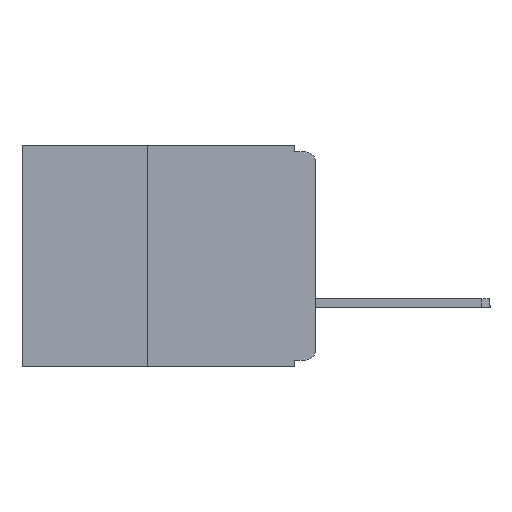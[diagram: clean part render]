
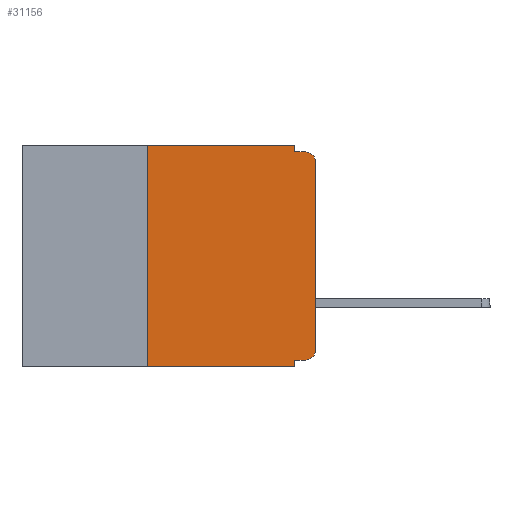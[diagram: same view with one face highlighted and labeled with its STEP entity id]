
A CAD part, left-side view. The second image highlights one B-rep face of the part: STEP entity #31156.
In plain terms, the highlighted planar face has unit normal (-1, 0, 0).
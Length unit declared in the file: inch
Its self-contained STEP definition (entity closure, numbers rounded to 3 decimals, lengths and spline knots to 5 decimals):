
#311 = VERTEX_POINT ( 'NONE', #29264 ) ;
#524 = DIRECTION ( 'NONE',  ( 0., 0., -1. ) ) ;
#1039 = ORIENTED_EDGE ( 'NONE', *, *, #28434, .F. ) ;
#1153 = VECTOR ( 'NONE', #16576, 39.37008 ) ;
#1636 = EDGE_CURVE ( 'NONE', #12275, #311, #32220, .T. ) ;
#1720 = LINE ( 'NONE', #27020, #27956 ) ;
#1995 = DIRECTION ( 'NONE',  ( -1., 0., 0. ) ) ;
#2628 = DIRECTION ( 'NONE',  ( 0., 0., -1. ) ) ;
#2970 = EDGE_CURVE ( 'NONE', #29224, #13932, #3359, .T. ) ;
#3237 = EDGE_CURVE ( 'NONE', #29224, #23874, #23327, .T. ) ;
#3359 = CIRCLE ( 'NONE', #26823, 0.015 ) ;
#4114 = LINE ( 'NONE', #27112, #16819 ) ;
#4340 = DIRECTION ( 'NONE',  ( 0., -1., 0. ) ) ;
#4427 = EDGE_CURVE ( 'NONE', #311, #22659, #15562, .T. ) ;
#4433 = ORIENTED_EDGE ( 'NONE', *, *, #3237, .F. ) ;
#5197 = VERTEX_POINT ( 'NONE', #29304 ) ;
#5385 = VECTOR ( 'NONE', #4340, 39.37008 ) ;
#5845 = CARTESIAN_POINT ( 'NONE',  ( 0., 0.437, 0. ) ) ;
#5871 = EDGE_CURVE ( 'NONE', #24997, #5197, #11295, .T. ) ;
#6599 = LINE ( 'NONE', #30603, #20154 ) ;
#8178 = CARTESIAN_POINT ( 'NONE',  ( 0., 0.25, -0.33 ) ) ;
#8509 = DIRECTION ( 'NONE',  ( 0., 1., 0. ) ) ;
#8709 = AXIS2_PLACEMENT_3D ( 'NONE', #32903, #16724, #524 ) ;
#8939 = VECTOR ( 'NONE', #8509, 39.37008 ) ;
#9753 = CARTESIAN_POINT ( 'NONE',  ( 0., 0.25, -0.33 ) ) ;
#9956 = ORIENTED_EDGE ( 'NONE', *, *, #15061, .T. ) ;
#9985 = ORIENTED_EDGE ( 'NONE', *, *, #2970, .T. ) ;
#11186 = CARTESIAN_POINT ( 'NONE',  ( 0., 0., -0.32 ) ) ;
#11295 = CIRCLE ( 'NONE', #8709, 0.015 ) ;
#12275 = VERTEX_POINT ( 'NONE', #9753 ) ;
#12284 = CARTESIAN_POINT ( 'NONE',  ( 0., 0.031, -0.32 ) ) ;
#12908 = DIRECTION ( 'NONE',  ( 0., -1., 0. ) ) ;
#13334 = ORIENTED_EDGE ( 'NONE', *, *, #4427, .F. ) ;
#13511 = DIRECTION ( 'NONE',  ( 0., 0., -1. ) ) ;
#13932 = VERTEX_POINT ( 'NONE', #15771 ) ;
#14404 = DIRECTION ( 'NONE',  ( 0., 0., 1. ) ) ;
#14422 = DIRECTION ( 'NONE',  ( 0., 0., 1. ) ) ;
#14890 = VERTEX_POINT ( 'NONE', #19896 ) ;
#15061 = EDGE_CURVE ( 'NONE', #12275, #25170, #18935, .T. ) ;
#15562 = LINE ( 'NONE', #5845, #1153 ) ;
#15644 = CARTESIAN_POINT ( 'NONE',  ( 0., 0., -0.025 ) ) ;
#15771 = CARTESIAN_POINT ( 'NONE',  ( 0., 0., -0.305 ) ) ;
#16576 = DIRECTION ( 'NONE',  ( 0., -1., 0. ) ) ;
#16724 = DIRECTION ( 'NONE',  ( -1., 0., 0. ) ) ;
#16819 = VECTOR ( 'NONE', #29806, 39.37008 ) ;
#17506 = VECTOR ( 'NONE', #12908, 39.37008 ) ;
#18240 = CARTESIAN_POINT ( 'NONE',  ( 0., 0.015, -0.305 ) ) ;
#18289 = FACE_OUTER_BOUND ( 'NONE', #19905, .T. ) ;
#18377 = LINE ( 'NONE', #21111, #17506 ) ;
#18566 = ORIENTED_EDGE ( 'NONE', *, *, #21559, .F. ) ;
#18868 = DIRECTION ( 'NONE',  ( 1., 0., 0. ) ) ;
#18935 = LINE ( 'NONE', #20583, #5385 ) ;
#19085 = CARTESIAN_POINT ( 'NONE',  ( 0., 0.031, -0.33 ) ) ;
#19896 = CARTESIAN_POINT ( 'NONE',  ( 0., 0.031, -0.01 ) ) ;
#19905 = EDGE_LOOP ( 'NONE', ( #29741, #32492, #1039, #18566, #13334, #25406, #9956, #29059, #4433, #9985 ) ) ;
#19943 = EDGE_CURVE ( 'NONE', #23874, #25170, #1720, .T. ) ;
#20154 = VECTOR ( 'NONE', #14404, 39.37008 ) ;
#20583 = CARTESIAN_POINT ( 'NONE',  ( 0., 0.437, -0.33 ) ) ;
#20972 = DIRECTION ( 'NONE',  ( 0., 0., -1. ) ) ;
#21111 = CARTESIAN_POINT ( 'NONE',  ( 0., 0., -0.01 ) ) ;
#21559 = EDGE_CURVE ( 'NONE', #22659, #14890, #4114, .T. ) ;
#22659 = VERTEX_POINT ( 'NONE', #34323 ) ;
#23327 = LINE ( 'NONE', #11186, #8939 ) ;
#23874 = VERTEX_POINT ( 'NONE', #12284 ) ;
#24997 = VERTEX_POINT ( 'NONE', #15644 ) ;
#25081 = VECTOR ( 'NONE', #14422, 39.37008 ) ;
#25170 = VERTEX_POINT ( 'NONE', #19085 ) ;
#25406 = ORIENTED_EDGE ( 'NONE', *, *, #1636, .F. ) ;
#26823 = AXIS2_PLACEMENT_3D ( 'NONE', #18240, #1995, #20972 ) ;
#27020 = CARTESIAN_POINT ( 'NONE',  ( 0., 0.031, -0.33 ) ) ;
#27112 = CARTESIAN_POINT ( 'NONE',  ( 0., 0.031, 0. ) ) ;
#27477 = EDGE_CURVE ( 'NONE', #13932, #24997, #6599, .T. ) ;
#27956 = VECTOR ( 'NONE', #13511, 39.37008 ) ;
#28434 = EDGE_CURVE ( 'NONE', #14890, #5197, #18377, .T. ) ;
#29059 = ORIENTED_EDGE ( 'NONE', *, *, #19943, .F. ) ;
#29224 = VERTEX_POINT ( 'NONE', #32465 ) ;
#29264 = CARTESIAN_POINT ( 'NONE',  ( 0., 0.25, 0. ) ) ;
#29304 = CARTESIAN_POINT ( 'NONE',  ( 0., 0.015, -0.01 ) ) ;
#29598 = PLANE ( 'NONE',  #30012 ) ;
#29741 = ORIENTED_EDGE ( 'NONE', *, *, #27477, .T. ) ;
#29806 = DIRECTION ( 'NONE',  ( 0., 0., -1. ) ) ;
#30012 = AXIS2_PLACEMENT_3D ( 'NONE', #34968, #18868, #2628 ) ;
#30603 = CARTESIAN_POINT ( 'NONE',  ( 0., 0., 0. ) ) ;
#31156 = ADVANCED_FACE ( 'NONE', ( #18289 ), #29598, .F. ) ;
#32220 = LINE ( 'NONE', #8178, #25081 ) ;
#32465 = CARTESIAN_POINT ( 'NONE',  ( 0., 0.015, -0.32 ) ) ;
#32492 = ORIENTED_EDGE ( 'NONE', *, *, #5871, .T. ) ;
#32903 = CARTESIAN_POINT ( 'NONE',  ( 0., 0.015, -0.025 ) ) ;
#34323 = CARTESIAN_POINT ( 'NONE',  ( 0., 0.031, 0. ) ) ;
#34968 = CARTESIAN_POINT ( 'NONE',  ( 0., 0.437, 0. ) ) ;
